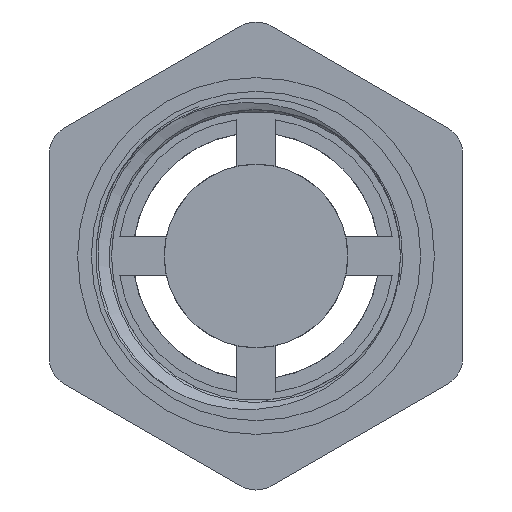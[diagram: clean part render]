
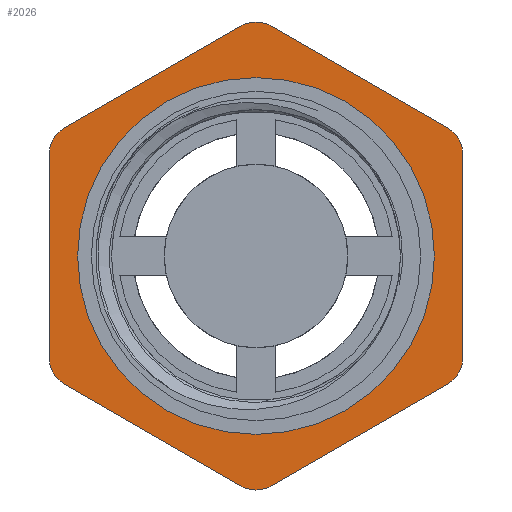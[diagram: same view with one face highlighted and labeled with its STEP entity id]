
A CAD part, front view. The second image highlights one B-rep face of the part: STEP entity #2026.
In plain terms, the highlighted planar face has unit normal (0, -1, 0).
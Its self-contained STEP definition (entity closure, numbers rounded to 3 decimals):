
#35=FACE_BOUND('',#269,.T.);
#65=PLANE('',#2237);
#160=FACE_OUTER_BOUND('',#268,.T.);
#268=EDGE_LOOP('',(#1675,#1676,#1677,#1678,#1679,#1680,#1681,#1682,#1683,
#1684,#1685,#1686));
#269=EDGE_LOOP('',(#1687));
#362=CIRCLE('',#2204,2.);
#370=CIRCLE('',#2217,2.);
#371=CIRCLE('',#2219,2.);
#372=CIRCLE('',#2222,2.);
#373=CIRCLE('',#2224,2.);
#374=CIRCLE('',#2227,2.);
#377=CIRCLE('',#2234,11.672);
#525=LINE('',#3810,#657);
#590=LINE('',#4209,#722);
#591=LINE('',#4211,#723);
#594=LINE('',#4226,#726);
#595=LINE('',#4227,#727);
#596=LINE('',#4228,#728);
#657=VECTOR('',#2428,10.);
#722=VECTOR('',#2695,10.);
#723=VECTOR('',#2698,10.);
#726=VECTOR('',#2717,10.);
#727=VECTOR('',#2718,10.);
#728=VECTOR('',#2719,10.);
#851=VERTEX_POINT('',#3807);
#852=VERTEX_POINT('',#3809);
#915=VERTEX_POINT('',#4159);
#919=VERTEX_POINT('',#4177);
#920=VERTEX_POINT('',#4178);
#921=VERTEX_POINT('',#4183);
#922=VERTEX_POINT('',#4184);
#923=VERTEX_POINT('',#4191);
#924=VERTEX_POINT('',#4192);
#925=VERTEX_POINT('',#4197);
#926=VERTEX_POINT('',#4198);
#927=VERTEX_POINT('',#4205);
#930=VERTEX_POINT('',#4219);
#1082=EDGE_CURVE('',#852,#851,#525,.T.);
#1189=EDGE_CURVE('',#852,#915,#362,.T.);
#1198=EDGE_CURVE('',#919,#920,#370,.T.);
#1201=EDGE_CURVE('',#921,#922,#371,.T.);
#1205=EDGE_CURVE('',#923,#924,#372,.T.);
#1208=EDGE_CURVE('',#925,#926,#373,.T.);
#1212=EDGE_CURVE('',#927,#851,#374,.T.);
#1214=EDGE_CURVE('',#919,#924,#590,.T.);
#1215=EDGE_CURVE('',#923,#915,#591,.T.);
#1219=EDGE_CURVE('',#930,#930,#377,.T.);
#1222=EDGE_CURVE('',#927,#926,#594,.T.);
#1223=EDGE_CURVE('',#925,#922,#595,.T.);
#1224=EDGE_CURVE('',#921,#920,#596,.T.);
#1675=ORIENTED_EDGE('',*,*,#1198,.F.);
#1676=ORIENTED_EDGE('',*,*,#1214,.T.);
#1677=ORIENTED_EDGE('',*,*,#1205,.F.);
#1678=ORIENTED_EDGE('',*,*,#1215,.T.);
#1679=ORIENTED_EDGE('',*,*,#1189,.F.);
#1680=ORIENTED_EDGE('',*,*,#1082,.T.);
#1681=ORIENTED_EDGE('',*,*,#1212,.F.);
#1682=ORIENTED_EDGE('',*,*,#1222,.T.);
#1683=ORIENTED_EDGE('',*,*,#1208,.F.);
#1684=ORIENTED_EDGE('',*,*,#1223,.T.);
#1685=ORIENTED_EDGE('',*,*,#1201,.F.);
#1686=ORIENTED_EDGE('',*,*,#1224,.T.);
#1687=ORIENTED_EDGE('',*,*,#1219,.T.);
#2026=ADVANCED_FACE('',(#160,#35),#65,.T.);
#2204=AXIS2_PLACEMENT_3D('',#4160,#2633,#2634);
#2217=AXIS2_PLACEMENT_3D('',#4179,#2660,#2661);
#2219=AXIS2_PLACEMENT_3D('',#4185,#2666,#2667);
#2222=AXIS2_PLACEMENT_3D('',#4193,#2675,#2676);
#2224=AXIS2_PLACEMENT_3D('',#4199,#2681,#2682);
#2227=AXIS2_PLACEMENT_3D('',#4206,#2690,#2691);
#2234=AXIS2_PLACEMENT_3D('',#4220,#2708,#2709);
#2237=AXIS2_PLACEMENT_3D('',#4225,#2715,#2716);
#2428=DIRECTION('',(0.,0.,1.));
#2633=DIRECTION('center_axis',(0.,1.,0.));
#2634=DIRECTION('ref_axis',(0.866,0.,-0.5));
#2660=DIRECTION('center_axis',(0.,1.,0.));
#2661=DIRECTION('ref_axis',(-0.866,0.,-0.5));
#2666=DIRECTION('center_axis',(0.,1.,0.));
#2667=DIRECTION('ref_axis',(-0.866,0.,0.5));
#2675=DIRECTION('center_axis',(0.,1.,0.));
#2676=DIRECTION('ref_axis',(0.,0.,-1.));
#2681=DIRECTION('center_axis',(0.,1.,0.));
#2682=DIRECTION('ref_axis',(0.,0.,1.));
#2690=DIRECTION('center_axis',(0.,1.,0.));
#2691=DIRECTION('ref_axis',(0.866,0.,0.5));
#2695=DIRECTION('',(0.866,0.,-0.5));
#2698=DIRECTION('',(0.866,0.,0.5));
#2708=DIRECTION('center_axis',(0.,1.,0.));
#2709=DIRECTION('ref_axis',(-1.,0.,0.));
#2715=DIRECTION('center_axis',(0.,-1.,0.));
#2716=DIRECTION('ref_axis',(0.,0.,-1.));
#2717=DIRECTION('',(-0.866,0.,0.5));
#2718=DIRECTION('',(-0.866,0.,-0.5));
#2719=DIRECTION('',(0.,0.,-1.));
#3807=CARTESIAN_POINT('',(13.524,-25.4,6.653));
#3809=CARTESIAN_POINT('',(13.524,-25.4,-6.653));
#3810=CARTESIAN_POINT('',(13.524,-25.4,-7.808));
#4159=CARTESIAN_POINT('',(12.524,-25.4,-8.385));
#4160=CARTESIAN_POINT('Origin',(11.524,-25.4,-6.653));
#4177=CARTESIAN_POINT('',(-12.524,-25.4,-8.385));
#4178=CARTESIAN_POINT('',(-13.524,-25.4,-6.653));
#4179=CARTESIAN_POINT('Origin',(-11.524,-25.4,-6.653));
#4183=CARTESIAN_POINT('',(-13.524,-25.4,6.653));
#4184=CARTESIAN_POINT('',(-12.524,-25.4,8.385));
#4185=CARTESIAN_POINT('Origin',(-11.524,-25.4,6.653));
#4191=CARTESIAN_POINT('',(1.,-25.4,-15.038));
#4192=CARTESIAN_POINT('',(-1.,-25.4,-15.038));
#4193=CARTESIAN_POINT('Origin',(0.,-25.4,-13.306));
#4197=CARTESIAN_POINT('',(-1.,-25.4,15.038));
#4198=CARTESIAN_POINT('',(1.,-25.4,15.038));
#4199=CARTESIAN_POINT('Origin',(0.,-25.4,13.306));
#4205=CARTESIAN_POINT('',(12.524,-25.4,8.385));
#4206=CARTESIAN_POINT('Origin',(11.524,-25.4,6.653));
#4209=CARTESIAN_POINT('',(-13.524,-25.4,-7.808));
#4211=CARTESIAN_POINT('',(0.,-25.4,-15.616));
#4219=CARTESIAN_POINT('',(11.672,-25.4,0.));
#4220=CARTESIAN_POINT('Origin',(0.,-25.4,0.));
#4225=CARTESIAN_POINT('Origin',(0.,-25.4,0.));
#4226=CARTESIAN_POINT('',(13.524,-25.4,7.808));
#4227=CARTESIAN_POINT('',(0.,-25.4,15.616));
#4228=CARTESIAN_POINT('',(-13.524,-25.4,7.808));
